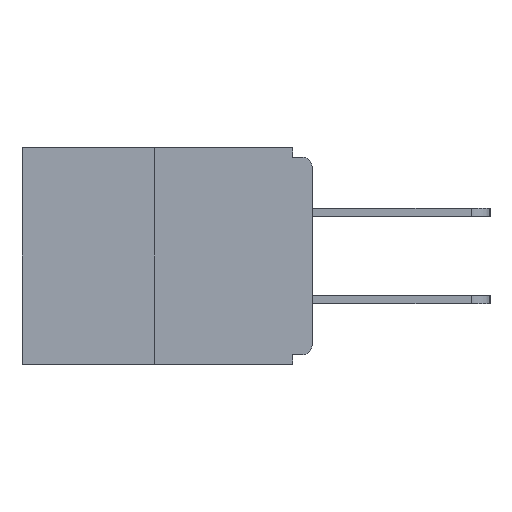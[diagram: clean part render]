
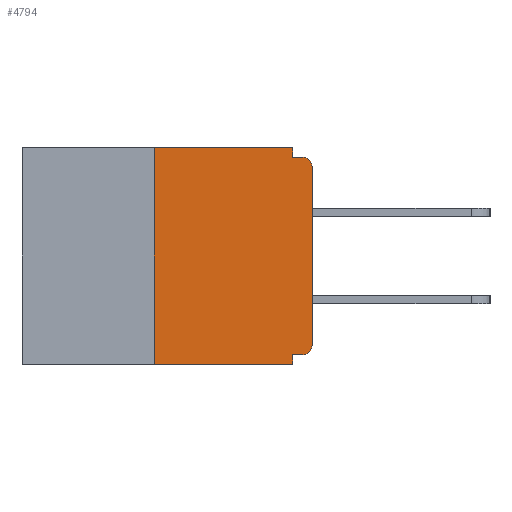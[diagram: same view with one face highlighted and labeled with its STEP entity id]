
A CAD part, left-side view. The second image highlights one B-rep face of the part: STEP entity #4794.
In plain terms, the highlighted planar face has unit normal (-1, 0, 0).
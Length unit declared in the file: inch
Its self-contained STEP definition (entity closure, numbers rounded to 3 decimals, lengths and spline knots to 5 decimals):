
#399 = CARTESIAN_POINT ( 'NONE',  ( 0., 0.015, -0.03 ) ) ;
#786 = CARTESIAN_POINT ( 'NONE',  ( 0., 0., -0.03 ) ) ;
#1313 = CARTESIAN_POINT ( 'NONE',  ( 0., 0.46, 0. ) ) ;
#2054 = CARTESIAN_POINT ( 'NONE',  ( 0., 0.46, 0. ) ) ;
#2083 = CARTESIAN_POINT ( 'NONE',  ( 0., 0.25, 0. ) ) ;
#2326 = ORIENTED_EDGE ( 'NONE', *, *, #19079, .F. ) ;
#2956 = EDGE_CURVE ( 'NONE', #8891, #17336, #15380, .T. ) ;
#3004 = AXIS2_PLACEMENT_3D ( 'NONE', #2054, #18914, #4876 ) ;
#3040 = DIRECTION ( 'NONE',  ( -1., 0., 0. ) ) ;
#3878 = VERTEX_POINT ( 'NONE', #17016 ) ;
#4347 = DIRECTION ( 'NONE',  ( 0., -1., 0. ) ) ;
#4540 = ORIENTED_EDGE ( 'NONE', *, *, #25451, .F. ) ;
#4658 = VECTOR ( 'NONE', #25184, 39.37008 ) ;
#4794 = ADVANCED_FACE ( 'NONE', ( #16576 ), #23986, .F. ) ;
#4876 = DIRECTION ( 'NONE',  ( 0., 0., -1. ) ) ;
#6005 = ORIENTED_EDGE ( 'NONE', *, *, #19945, .T. ) ;
#6695 = DIRECTION ( 'NONE',  ( 0., 0., -1. ) ) ;
#6797 = CARTESIAN_POINT ( 'NONE',  ( 0., 0.015, -0.313 ) ) ;
#6811 = VERTEX_POINT ( 'NONE', #14016 ) ;
#7383 = LINE ( 'NONE', #9231, #13812 ) ;
#7454 = ORIENTED_EDGE ( 'NONE', *, *, #15023, .F. ) ;
#7670 = CARTESIAN_POINT ( 'NONE',  ( 0., 0., 0. ) ) ;
#8564 = DIRECTION ( 'NONE',  ( 0., -1., 0. ) ) ;
#8848 = AXIS2_PLACEMENT_3D ( 'NONE', #399, #3040, #26988 ) ;
#8891 = VERTEX_POINT ( 'NONE', #9219 ) ;
#8999 = VECTOR ( 'NONE', #9371, 39.37008 ) ;
#9066 = CARTESIAN_POINT ( 'NONE',  ( 0., 0.031, 0. ) ) ;
#9219 = CARTESIAN_POINT ( 'NONE',  ( 0., 0.031, 0. ) ) ;
#9231 = CARTESIAN_POINT ( 'NONE',  ( 0., 0.46, -0.343 ) ) ;
#9371 = DIRECTION ( 'NONE',  ( 0., 0., -1. ) ) ;
#10196 = ORIENTED_EDGE ( 'NONE', *, *, #10900, .T. ) ;
#10900 = EDGE_CURVE ( 'NONE', #22355, #24519, #23851, .T. ) ;
#10981 = VECTOR ( 'NONE', #24505, 39.37008 ) ;
#12478 = VECTOR ( 'NONE', #8564, 39.37008 ) ;
#13812 = VECTOR ( 'NONE', #31105, 39.37008 ) ;
#13848 = EDGE_CURVE ( 'NONE', #6811, #17066, #7383, .T. ) ;
#14016 = CARTESIAN_POINT ( 'NONE',  ( 0., 0.25, -0.343 ) ) ;
#14294 = CARTESIAN_POINT ( 'NONE',  ( 0., 0., -0.328 ) ) ;
#15023 = EDGE_CURVE ( 'NONE', #17336, #28268, #27296, .T. ) ;
#15327 = CIRCLE ( 'NONE', #26558, 0.015 ) ;
#15380 = LINE ( 'NONE', #9066, #8999 ) ;
#16576 = FACE_OUTER_BOUND ( 'NONE', #22652, .T. ) ;
#16597 = CARTESIAN_POINT ( 'NONE',  ( 0., 0.031, -0.343 ) ) ;
#16912 = CARTESIAN_POINT ( 'NONE',  ( 0., 0.031, -0.328 ) ) ;
#17016 = CARTESIAN_POINT ( 'NONE',  ( 0., 0.25, 0. ) ) ;
#17066 = VERTEX_POINT ( 'NONE', #16597 ) ;
#17183 = LINE ( 'NONE', #14294, #27010 ) ;
#17336 = VERTEX_POINT ( 'NONE', #25040 ) ;
#17740 = CARTESIAN_POINT ( 'NONE',  ( 0., 0.015, -0.328 ) ) ;
#18007 = EDGE_CURVE ( 'NONE', #20670, #29654, #17183, .T. ) ;
#18914 = DIRECTION ( 'NONE',  ( 1., 0., 0. ) ) ;
#18938 = DIRECTION ( 'NONE',  ( 0., 0., 1. ) ) ;
#18951 = ORIENTED_EDGE ( 'NONE', *, *, #2956, .F. ) ;
#19079 = EDGE_CURVE ( 'NONE', #29654, #17066, #26227, .T. ) ;
#19945 = EDGE_CURVE ( 'NONE', #24519, #28268, #29173, .T. ) ;
#20670 = VERTEX_POINT ( 'NONE', #17740 ) ;
#20688 = CARTESIAN_POINT ( 'NONE',  ( 0., 0., -0.313 ) ) ;
#20733 = EDGE_CURVE ( 'NONE', #3878, #8891, #21550, .T. ) ;
#21550 = LINE ( 'NONE', #1313, #12478 ) ;
#21691 = ORIENTED_EDGE ( 'NONE', *, *, #18007, .F. ) ;
#22355 = VERTEX_POINT ( 'NONE', #20688 ) ;
#22652 = EDGE_LOOP ( 'NONE', ( #30884, #4540, #25750, #2326, #21691, #30153, #10196, #6005, #7454, #18951 ) ) ;
#22957 = CARTESIAN_POINT ( 'NONE',  ( 0., 0.031, -0.343 ) ) ;
#23247 = EDGE_CURVE ( 'NONE', #20670, #22355, #15327, .T. ) ;
#23851 = LINE ( 'NONE', #7670, #10981 ) ;
#23986 = PLANE ( 'NONE',  #3004 ) ;
#24505 = DIRECTION ( 'NONE',  ( 0., 0., 1. ) ) ;
#24519 = VERTEX_POINT ( 'NONE', #786 ) ;
#25040 = CARTESIAN_POINT ( 'NONE',  ( 0., 0.031, -0.015 ) ) ;
#25184 = DIRECTION ( 'NONE',  ( 0., 0., -1. ) ) ;
#25451 = EDGE_CURVE ( 'NONE', #6811, #3878, #27756, .T. ) ;
#25486 = CARTESIAN_POINT ( 'NONE',  ( 0., 0., -0.015 ) ) ;
#25750 = ORIENTED_EDGE ( 'NONE', *, *, #13848, .T. ) ;
#26064 = DIRECTION ( 'NONE',  ( -1., 0., 0. ) ) ;
#26227 = LINE ( 'NONE', #22957, #4658 ) ;
#26558 = AXIS2_PLACEMENT_3D ( 'NONE', #6797, #26064, #6695 ) ;
#26988 = DIRECTION ( 'NONE',  ( 0., 0., -1. ) ) ;
#27010 = VECTOR ( 'NONE', #31204, 39.37008 ) ;
#27296 = LINE ( 'NONE', #25486, #27326 ) ;
#27326 = VECTOR ( 'NONE', #4347, 39.37008 ) ;
#27756 = LINE ( 'NONE', #2083, #31157 ) ;
#28268 = VERTEX_POINT ( 'NONE', #29851 ) ;
#29173 = CIRCLE ( 'NONE', #8848, 0.015 ) ;
#29654 = VERTEX_POINT ( 'NONE', #16912 ) ;
#29851 = CARTESIAN_POINT ( 'NONE',  ( 0., 0.015, -0.015 ) ) ;
#30153 = ORIENTED_EDGE ( 'NONE', *, *, #23247, .T. ) ;
#30884 = ORIENTED_EDGE ( 'NONE', *, *, #20733, .F. ) ;
#31105 = DIRECTION ( 'NONE',  ( 0., -1., 0. ) ) ;
#31157 = VECTOR ( 'NONE', #18938, 39.37008 ) ;
#31204 = DIRECTION ( 'NONE',  ( 0., 1., 0. ) ) ;
